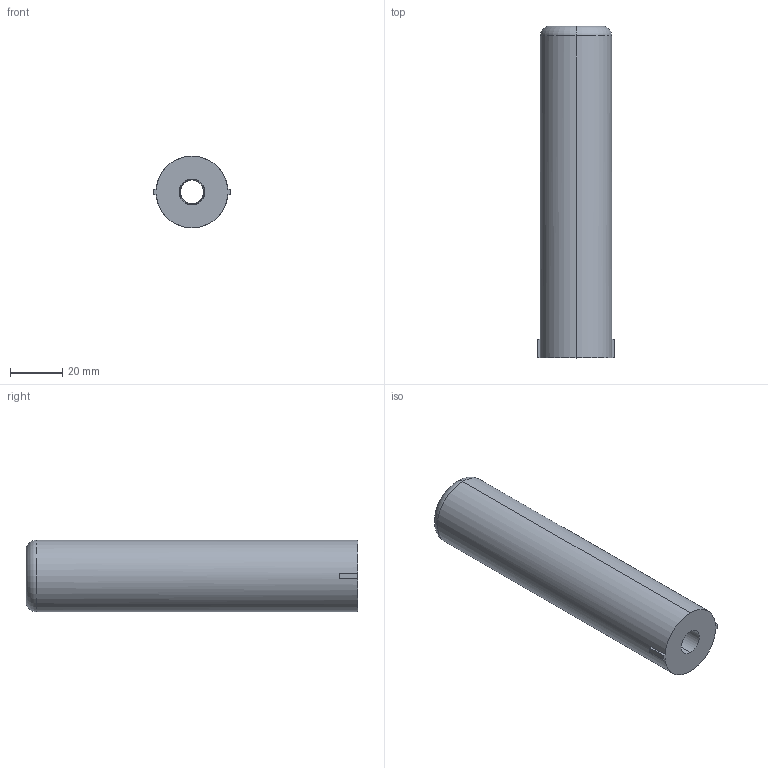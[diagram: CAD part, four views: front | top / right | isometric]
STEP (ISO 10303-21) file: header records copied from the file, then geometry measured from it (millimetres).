
FILE_DESCRIPTION (( 'STEP AP214' ), '1' );
FILE_NAME ('380_barrel.STEP', '2013-10-23T01:44:51', ( '' ), ( '' ), 'SwSTEP 2.0', 'SolidWorks 2013', '' );
FILE_SCHEMA (( 'AUTOMOTIVE_DESIGN' ));
Length unit declared in the file: inch
Products named in the file (1): 380_barrel
Bounding box: 29.46 x 127 x 27.43 mm (x, y, z)
Volume: 65153.4 mm3; surface area: 16994 mm2
Topology: 1 solids, 1 shells, 85 faces, 225 edges, 142 vertices
Faces by surface type: bspline 30, cylinder 22, plane 20, torus 13
Entity records: 6860 total; most frequent: CARTESIAN_POINT 5037, ORIENTED_EDGE 450, DIRECTION 296, EDGE_CURVE 225, VERTEX_POINT 142, AXIS2_PLACEMENT_3D 117, EDGE_LOOP 87, ADVANCED_FACE 85
